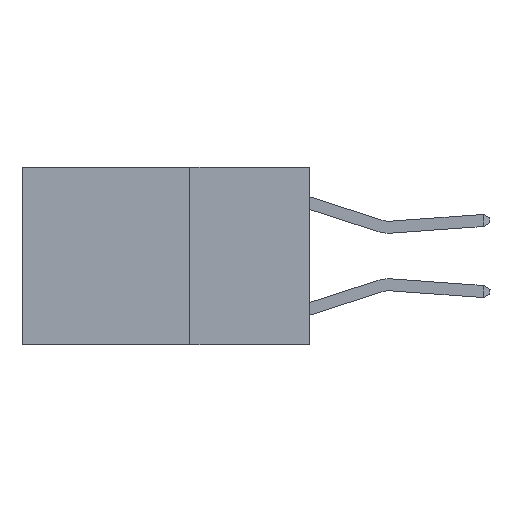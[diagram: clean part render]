
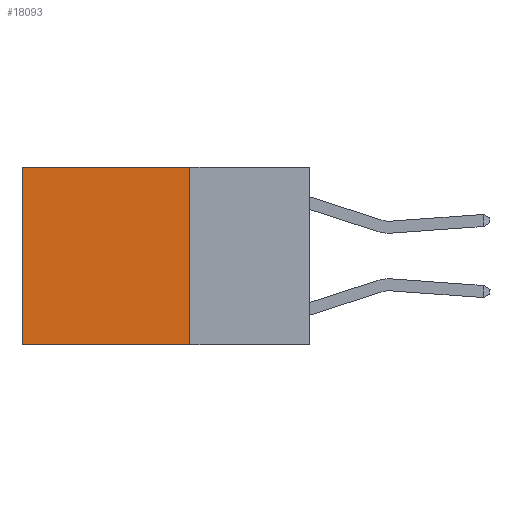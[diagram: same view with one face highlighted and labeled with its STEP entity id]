
A CAD part, left-side view. The second image highlights one B-rep face of the part: STEP entity #18093.
In plain terms, the highlighted planar face has unit normal (-1, 0, 0).
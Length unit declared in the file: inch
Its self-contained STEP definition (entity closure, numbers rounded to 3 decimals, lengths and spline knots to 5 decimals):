
#1500 = VERTEX_POINT ( 'NONE', #19926 ) ;
#1817 = CARTESIAN_POINT ( 'NONE',  ( 0.2625, 0.25, 0. ) ) ;
#2359 = ORIENTED_EDGE ( 'NONE', *, *, #11279, .F. ) ;
#2977 = CARTESIAN_POINT ( 'NONE',  ( 0.2625, 0.6, 0. ) ) ;
#3750 = VERTEX_POINT ( 'NONE', #2977 ) ;
#3842 = DIRECTION ( 'NONE',  ( 0., 1., 0. ) ) ;
#4532 = FACE_OUTER_BOUND ( 'NONE', #20831, .T. ) ;
#5708 = ORIENTED_EDGE ( 'NONE', *, *, #15686, .F. ) ;
#6055 = CARTESIAN_POINT ( 'NONE',  ( 0.2625, 0.25, -0.37 ) ) ;
#6274 = DIRECTION ( 'NONE',  ( 1., 0., 0. ) ) ;
#7495 = VECTOR ( 'NONE', #12653, 39.37008 ) ;
#8783 = VECTOR ( 'NONE', #24733, 39.37008 ) ;
#10440 = LINE ( 'NONE', #26125, #26809 ) ;
#10535 = VERTEX_POINT ( 'NONE', #14134 ) ;
#11279 = EDGE_CURVE ( 'NONE', #13894, #1500, #16315, .T. ) ;
#11328 = EDGE_CURVE ( 'NONE', #10535, #3750, #10440, .T. ) ;
#11393 = CARTESIAN_POINT ( 'NONE',  ( 0.2625, 0.25, 0. ) ) ;
#12653 = DIRECTION ( 'NONE',  ( 0., 0., -1. ) ) ;
#13286 = LINE ( 'NONE', #11393, #8783 ) ;
#13522 = ORIENTED_EDGE ( 'NONE', *, *, #11328, .T. ) ;
#13894 = VERTEX_POINT ( 'NONE', #26102 ) ;
#14134 = CARTESIAN_POINT ( 'NONE',  ( 0.2625, 0.25, 0. ) ) ;
#14239 = ORIENTED_EDGE ( 'NONE', *, *, #27664, .T. ) ;
#15686 = EDGE_CURVE ( 'NONE', #10535, #13894, #13286, .T. ) ;
#16315 = LINE ( 'NONE', #6055, #27502 ) ;
#17749 = AXIS2_PLACEMENT_3D ( 'NONE', #1817, #6274, #21759 ) ;
#18093 = ADVANCED_FACE ( 'NONE', ( #4532 ), #19529, .F. ) ;
#19291 = LINE ( 'NONE', #28238, #7495 ) ;
#19529 = PLANE ( 'NONE',  #17749 ) ;
#19926 = CARTESIAN_POINT ( 'NONE',  ( 0.2625, 0.6, -0.37 ) ) ;
#20831 = EDGE_LOOP ( 'NONE', ( #14239, #2359, #5708, #13522 ) ) ;
#21759 = DIRECTION ( 'NONE',  ( 0., 0., -1. ) ) ;
#24733 = DIRECTION ( 'NONE',  ( 0., 0., -1. ) ) ;
#26102 = CARTESIAN_POINT ( 'NONE',  ( 0.2625, 0.25, -0.37 ) ) ;
#26125 = CARTESIAN_POINT ( 'NONE',  ( 0.2625, 0.25, 0. ) ) ;
#26809 = VECTOR ( 'NONE', #28366, 39.37008 ) ;
#27502 = VECTOR ( 'NONE', #3842, 39.37008 ) ;
#27664 = EDGE_CURVE ( 'NONE', #3750, #1500, #19291, .T. ) ;
#28238 = CARTESIAN_POINT ( 'NONE',  ( 0.2625, 0.6, 0. ) ) ;
#28366 = DIRECTION ( 'NONE',  ( 0., 1., 0. ) ) ;
